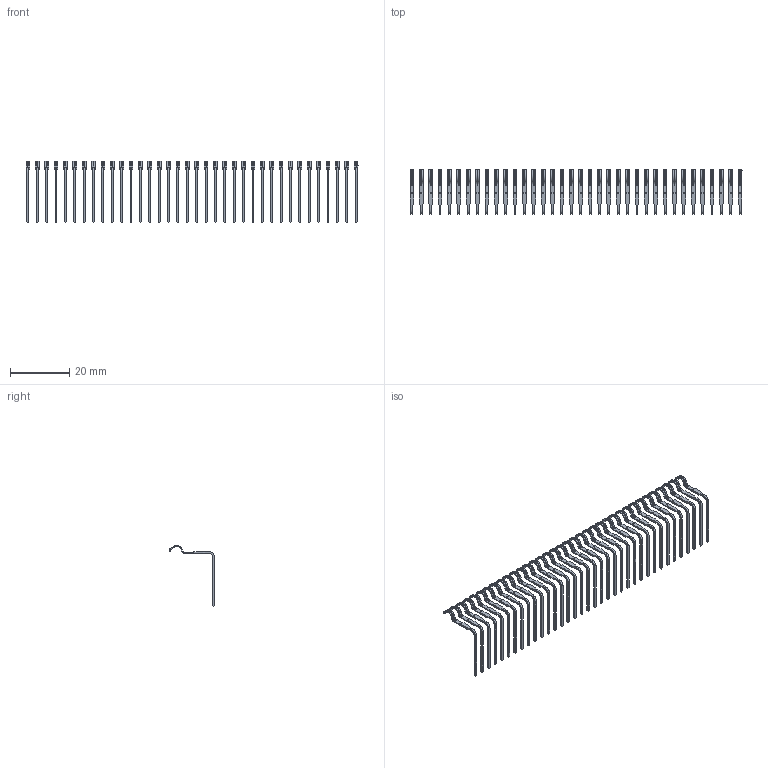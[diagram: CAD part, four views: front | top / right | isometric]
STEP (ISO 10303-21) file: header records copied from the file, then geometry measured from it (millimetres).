
FILE_DESCRIPTION (( 'STEP AP203' ), '1' );
FILE_NAME ('346-036-559-102.STEP', '2022-05-07T01:41:54', ( '' ), ( '' ), 'SwSTEP 2.0', 'SolidWorks 2020', '' );
FILE_SCHEMA (( 'CONFIG_CONTROL_DESIGN' ));
Length unit declared in the file: inch
Products named in the file (3): 346-036-559-102; 346 Part_Flush Mounting Lugs - 0.128 Dia; 345-292-001_558 559 Tail - 1
Assembly tree (37 placements, depth 2):
  346-036-559-102
    346 Part_Flush Mounting Lugs - 0.128 Dia
    345-292-001_558 559 Tail - 1  x36
Bounding box: 112.39 x 15.18 x 20.67 mm (x, y, z)
Volume: 531.6 mm3; surface area: 3595.3 mm2
Topology: 36 solids, 36 shells, 1728 faces, 5040 edges, 3312 vertices
Faces by surface type: plane 1152, cylinder 576
Entity records: 23237 total; most frequent: CARTESIAN_POINT 3992, ORIENTED_EDGE 3962, DIRECTION 3529, EDGE_CURVE 1981, VECTOR 1705, LINE 1705, VERTEX_POINT 1318, AXIS2_PLACEMENT_3D 912
